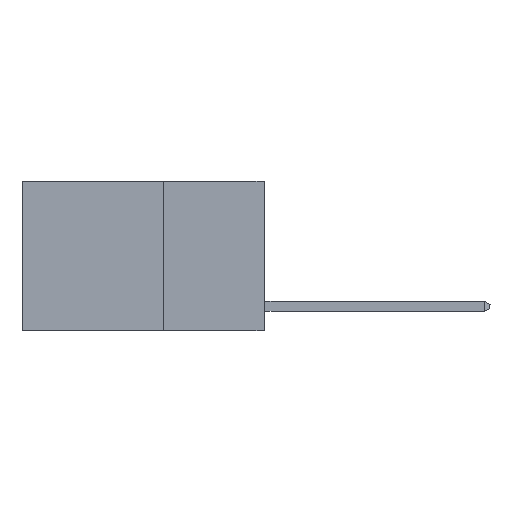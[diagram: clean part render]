
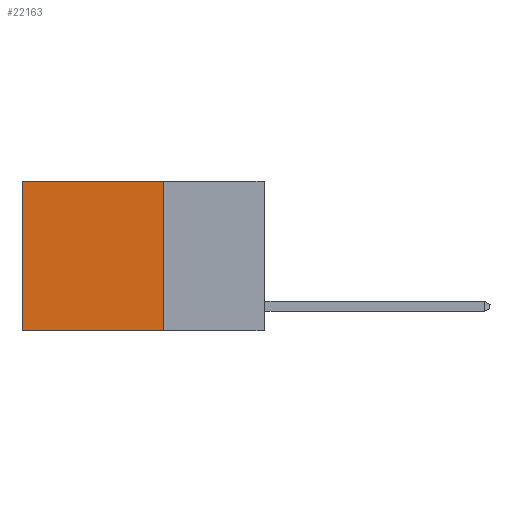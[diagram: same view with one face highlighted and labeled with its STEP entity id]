
A CAD part, left-side view. The second image highlights one B-rep face of the part: STEP entity #22163.
In plain terms, the highlighted planar face has unit normal (-1, 0, 0).
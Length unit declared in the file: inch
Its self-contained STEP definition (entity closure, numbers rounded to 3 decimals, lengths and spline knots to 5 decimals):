
#196 = FACE_OUTER_BOUND ( 'NONE', #2175, .T. ) ;
#762 = LINE ( 'NONE', #1609, #20398 ) ;
#816 = LINE ( 'NONE', #6433, #20455 ) ;
#1609 = CARTESIAN_POINT ( 'NONE',  ( 0.2625, 0.6, 0. ) ) ;
#2175 = EDGE_LOOP ( 'NONE', ( #14849, #23098, #13010, #21239 ) ) ;
#2323 = DIRECTION ( 'NONE',  ( 0., 1., 0. ) ) ;
#4297 = VECTOR ( 'NONE', #6614, 39.37008 ) ;
#4679 = LINE ( 'NONE', #13690, #19236 ) ;
#5331 = CARTESIAN_POINT ( 'NONE',  ( 0.2625, 0.25, 0. ) ) ;
#6433 = CARTESIAN_POINT ( 'NONE',  ( 0.2625, 0.25, -0.37 ) ) ;
#6614 = DIRECTION ( 'NONE',  ( 0., 0., -1. ) ) ;
#7265 = DIRECTION ( 'NONE',  ( 0., 0., -1. ) ) ;
#9340 = LINE ( 'NONE', #10415, #4297 ) ;
#9642 = VERTEX_POINT ( 'NONE', #11080 ) ;
#9992 = VERTEX_POINT ( 'NONE', #14415 ) ;
#10415 = CARTESIAN_POINT ( 'NONE',  ( 0.2625, 0.25, 0. ) ) ;
#11080 = CARTESIAN_POINT ( 'NONE',  ( 0.2625, 0.25, -0.37 ) ) ;
#12382 = EDGE_CURVE ( 'NONE', #9642, #9992, #816, .T. ) ;
#12935 = EDGE_CURVE ( 'NONE', #16977, #20625, #4679, .T. ) ;
#13010 = ORIENTED_EDGE ( 'NONE', *, *, #14435, .F. ) ;
#13690 = CARTESIAN_POINT ( 'NONE',  ( 0.2625, 0.25, 0. ) ) ;
#14415 = CARTESIAN_POINT ( 'NONE',  ( 0.2625, 0.6, -0.37 ) ) ;
#14435 = EDGE_CURVE ( 'NONE', #16977, #9642, #9340, .T. ) ;
#14849 = ORIENTED_EDGE ( 'NONE', *, *, #23426, .T. ) ;
#15860 = CARTESIAN_POINT ( 'NONE',  ( 0.2625, 0.25, 0. ) ) ;
#16732 = PLANE ( 'NONE',  #23841 ) ;
#16977 = VERTEX_POINT ( 'NONE', #15860 ) ;
#18650 = DIRECTION ( 'NONE',  ( 1., 0., 0. ) ) ;
#18756 = DIRECTION ( 'NONE',  ( 0., 0., -1. ) ) ;
#19236 = VECTOR ( 'NONE', #2323, 39.37008 ) ;
#20398 = VECTOR ( 'NONE', #18756, 39.37008 ) ;
#20455 = VECTOR ( 'NONE', #23521, 39.37008 ) ;
#20625 = VERTEX_POINT ( 'NONE', #21877 ) ;
#21239 = ORIENTED_EDGE ( 'NONE', *, *, #12935, .T. ) ;
#21877 = CARTESIAN_POINT ( 'NONE',  ( 0.2625, 0.6, 0. ) ) ;
#22163 = ADVANCED_FACE ( 'NONE', ( #196 ), #16732, .F. ) ;
#23098 = ORIENTED_EDGE ( 'NONE', *, *, #12382, .F. ) ;
#23426 = EDGE_CURVE ( 'NONE', #20625, #9992, #762, .T. ) ;
#23521 = DIRECTION ( 'NONE',  ( 0., 1., 0. ) ) ;
#23841 = AXIS2_PLACEMENT_3D ( 'NONE', #5331, #18650, #7265 ) ;
